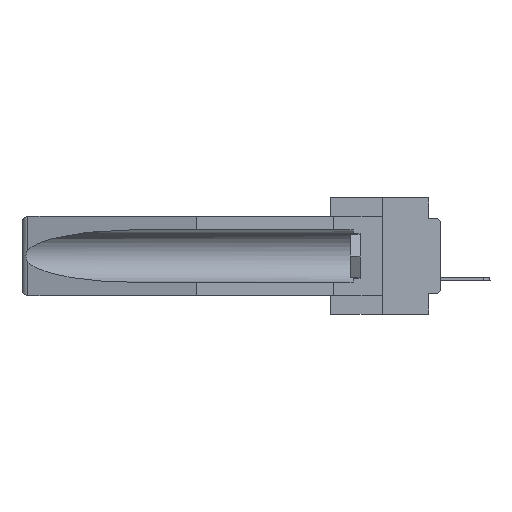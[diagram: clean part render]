
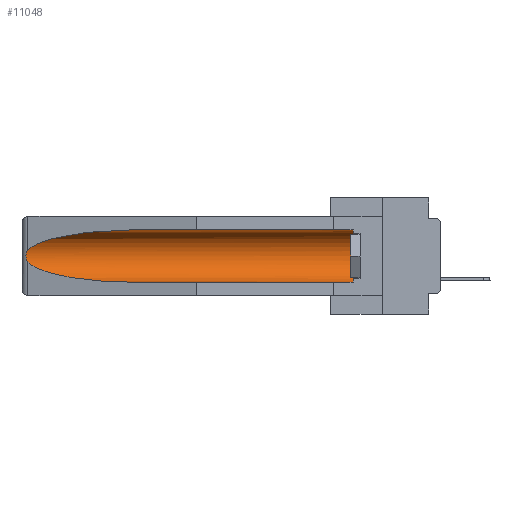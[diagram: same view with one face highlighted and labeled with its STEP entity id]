
A CAD part, left-side view. The second image highlights one B-rep face of the part: STEP entity #11048.
In plain terms, the highlighted cylindrical face has radius 2.857 mm (diameter 5.715 mm), a partial arc.
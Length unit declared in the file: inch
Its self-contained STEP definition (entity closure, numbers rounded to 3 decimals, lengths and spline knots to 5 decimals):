
#915 = CARTESIAN_POINT ( 'NONE',  ( 0.155, 1.07973, -0.059 ) ) ;
#962 = EDGE_CURVE ( 'NONE', #7308, #8460, #22255, .T. ) ;
#1354 = VERTEX_POINT ( 'NONE', #15227 ) ;
#1407 = CARTESIAN_POINT ( 'NONE',  ( 0.155, -0.30754, -0.059 ) ) ;
#1490 = EDGE_CURVE ( 'NONE', #5657, #1354, #9482, .T. ) ;
#2023 = AXIS2_PLACEMENT_3D ( 'NONE', #9337, #17874, #26511 ) ;
#2044 = VERTEX_POINT ( 'NONE', #13852 ) ;
#2657 = CARTESIAN_POINT ( 'NONE',  ( 0.21114, 1.30732, -0.284 ) ) ;
#5657 = VERTEX_POINT ( 'NONE', #27759 ) ;
#5896 = CARTESIAN_POINT ( 'NONE',  ( 0.26537, 1.52718, -0.19328 ) ) ;
#6193 = VERTEX_POINT ( 'NONE', #5896 ) ;
#6326 = EDGE_CURVE ( 'NONE', #6193, #2044, #19963, .T. ) ;
#6718 = CARTESIAN_POINT ( 'NONE',  ( 0.2673, 1.53269, -0.17917 ) ) ;
#7027 = CARTESIAN_POINT ( 'NONE',  ( 0.155, -0.30754, -0.1715 ) ) ;
#7308 = VERTEX_POINT ( 'NONE', #915 ) ;
#7722 = DIRECTION ( 'NONE',  ( 0., 1., 0. ) ) ;
#8460 = VERTEX_POINT ( 'NONE', #12602 ) ;
#8748 = ORIENTED_EDGE ( 'NONE', *, *, #1490, .T. ) ;
#9104 = CARTESIAN_POINT ( 'NONE',  ( 0.25451, 1.48313, -0.24835 ) ) ;
#9337 = CARTESIAN_POINT ( 'NONE',  ( 0.155, 0.126, -0.1715 ) ) ;
#9394 = ORIENTED_EDGE ( 'NONE', *, *, #23267, .T. ) ;
#9482 = CIRCLE ( 'NONE', #2023, 0.1125 ) ;
#10455 = CARTESIAN_POINT ( 'NONE',  ( 0.21114, 1.30732, -0.059 ) ) ;
#10984 = CARTESIAN_POINT ( 'NONE',  ( 0.2675, 1.53308, -0.17534 ) ) ;
#11048 = ADVANCED_FACE ( 'NONE', ( #24506 ), #27114, .F. ) ;
#11947 = B_SPLINE_CURVE_WITH_KNOTS ( 'NONE', 3,
 ( #21837, #17606, #28578, #26793, #13195, #10984, #6718, #19918, #17740, #26659 ),
 .UNSPECIFIED., .F., .F.,
 ( 4, 2, 2, 2, 4 ),
 ( 0., 0.00029, 0.00058, 0.00087, 0.00117 ),
 .UNSPECIFIED. ) ;
#12231 = CARTESIAN_POINT ( 'NONE',  ( 0.155, 1.07973, -0.059 ) ) ;
#12602 = CARTESIAN_POINT ( 'NONE',  ( 0.26537, 1.52718, -0.14972 ) ) ;
#12687 = VECTOR ( 'NONE', #7722, 39.37008 ) ;
#12823 = CARTESIAN_POINT ( 'NONE',  ( 0.26537, 1.52718, -0.14972 ) ) ;
#13195 = CARTESIAN_POINT ( 'NONE',  ( 0.2675, 1.53308, -0.16763 ) ) ;
#13852 = CARTESIAN_POINT ( 'NONE',  ( 0.155, 1.07973, -0.284 ) ) ;
#15227 = CARTESIAN_POINT ( 'NONE',  ( 0.155, 0.126, -0.059 ) ) ;
#15975 = DIRECTION ( 'NONE',  ( 0., 1., 0. ) ) ;
#16293 = EDGE_CURVE ( 'NONE', #5657, #2044, #18611, .T. ) ;
#16646 = LINE ( 'NONE', #1407, #12687 ) ;
#16776 = ORIENTED_EDGE ( 'NONE', *, *, #25166, .T. ) ;
#17606 = CARTESIAN_POINT ( 'NONE',  ( 0.26597, 1.52961, -0.15275 ) ) ;
#17643 = DIRECTION ( 'NONE',  ( 0., 0., 1. ) ) ;
#17740 = CARTESIAN_POINT ( 'NONE',  ( 0.26597, 1.5296, -0.19026 ) ) ;
#17874 = DIRECTION ( 'NONE',  ( 0., -1., 0. ) ) ;
#18050 = VECTOR ( 'NONE', #21099, 39.37008 ) ;
#18611 = LINE ( 'NONE', #25216, #18050 ) ;
#19918 = CARTESIAN_POINT ( 'NONE',  ( 0.26655, 1.53094, -0.18657 ) ) ;
#19963 =( BOUNDED_CURVE ( )  B_SPLINE_CURVE ( 3, ( #22166, #9104, #2657, #20229 ),
 .UNSPECIFIED., .F., .F. ) 
 B_SPLINE_CURVE_WITH_KNOTS ( ( 4, 4 ),
 ( 0.1948, 1.5708 ),
 .UNSPECIFIED. ) 
 CURVE ( )  GEOMETRIC_REPRESENTATION_ITEM ( )  RATIONAL_B_SPLINE_CURVE ( ( 1., 0.848, 0.848, 1. ) ) 
 REPRESENTATION_ITEM ( '' )  );
#20229 = CARTESIAN_POINT ( 'NONE',  ( 0.155, 1.07973, -0.284 ) ) ;
#20327 = EDGE_LOOP ( 'NONE', ( #27896, #16776, #27194, #28302, #8748, #9394 ) ) ;
#21099 = DIRECTION ( 'NONE',  ( 0., 1., 0. ) ) ;
#21837 = CARTESIAN_POINT ( 'NONE',  ( 0.26537, 1.52718, -0.14972 ) ) ;
#22166 = CARTESIAN_POINT ( 'NONE',  ( 0.26537, 1.52718, -0.19328 ) ) ;
#22255 =( BOUNDED_CURVE ( )  B_SPLINE_CURVE ( 3, ( #12231, #10455, #27900, #12823 ),
 .UNSPECIFIED., .F., .F. ) 
 B_SPLINE_CURVE_WITH_KNOTS ( ( 4, 4 ),
 ( 4.71239, 6.08839 ),
 .UNSPECIFIED. ) 
 CURVE ( )  GEOMETRIC_REPRESENTATION_ITEM ( )  RATIONAL_B_SPLINE_CURVE ( ( 1., 0.848, 0.848, 1. ) ) 
 REPRESENTATION_ITEM ( '' )  );
#23267 = EDGE_CURVE ( 'NONE', #1354, #7308, #16646, .T. ) ;
#24506 = FACE_OUTER_BOUND ( 'NONE', #20327, .T. ) ;
#25166 = EDGE_CURVE ( 'NONE', #8460, #6193, #11947, .T. ) ;
#25216 = CARTESIAN_POINT ( 'NONE',  ( 0.155, -0.30754, -0.284 ) ) ;
#25826 = AXIS2_PLACEMENT_3D ( 'NONE', #7027, #15975, #17643 ) ;
#26511 = DIRECTION ( 'NONE',  ( 0., 0., 1. ) ) ;
#26659 = CARTESIAN_POINT ( 'NONE',  ( 0.26537, 1.52718, -0.19328 ) ) ;
#26793 = CARTESIAN_POINT ( 'NONE',  ( 0.2673, 1.5327, -0.16383 ) ) ;
#27114 = CYLINDRICAL_SURFACE ( 'NONE', #25826, 0.1125 ) ;
#27194 = ORIENTED_EDGE ( 'NONE', *, *, #6326, .T. ) ;
#27759 = CARTESIAN_POINT ( 'NONE',  ( 0.155, 0.126, -0.284 ) ) ;
#27896 = ORIENTED_EDGE ( 'NONE', *, *, #962, .T. ) ;
#27900 = CARTESIAN_POINT ( 'NONE',  ( 0.25451, 1.48313, -0.09465 ) ) ;
#28302 = ORIENTED_EDGE ( 'NONE', *, *, #16293, .F. ) ;
#28578 = CARTESIAN_POINT ( 'NONE',  ( 0.26654, 1.53092, -0.15636 ) ) ;
